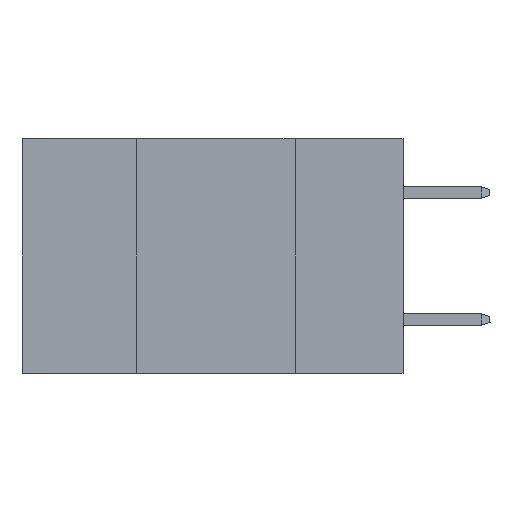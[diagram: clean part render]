
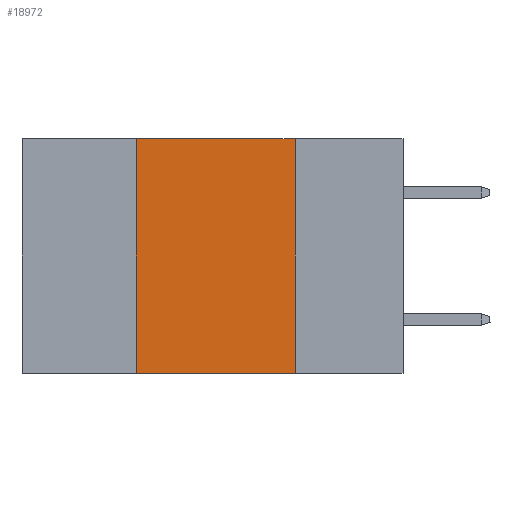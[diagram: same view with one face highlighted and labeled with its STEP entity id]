
A CAD part, left-side view. The second image highlights one B-rep face of the part: STEP entity #18972.
In plain terms, the highlighted planar face has unit normal (-1, 0, 0).
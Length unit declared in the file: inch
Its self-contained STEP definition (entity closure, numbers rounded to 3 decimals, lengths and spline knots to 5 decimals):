
#32 = FACE_OUTER_BOUND ( 'NONE', #22757, .T. ) ;
#1107 = LINE ( 'NONE', #20510, #4530 ) ;
#1899 = VECTOR ( 'NONE', #18962, 39.37008 ) ;
#3018 = VERTEX_POINT ( 'NONE', #8340 ) ;
#3352 = DIRECTION ( 'NONE',  ( 0., 0., 1. ) ) ;
#3910 = PLANE ( 'NONE',  #14600 ) ;
#4316 = ORIENTED_EDGE ( 'NONE', *, *, #20041, .F. ) ;
#4329 = ORIENTED_EDGE ( 'NONE', *, *, #23785, .F. ) ;
#4530 = VECTOR ( 'NONE', #3352, 39.37008 ) ;
#4694 = ORIENTED_EDGE ( 'NONE', *, *, #9097, .T. ) ;
#5408 = VERTEX_POINT ( 'NONE', #8765 ) ;
#5969 = LINE ( 'NONE', #8219, #9829 ) ;
#6471 = EDGE_CURVE ( 'NONE', #5408, #3018, #1107, .T. ) ;
#7242 = VECTOR ( 'NONE', #10525, 39.37008 ) ;
#7670 = CARTESIAN_POINT ( 'NONE',  ( 0., 0.6, 0. ) ) ;
#8219 = CARTESIAN_POINT ( 'NONE',  ( 0., 0.6, 0. ) ) ;
#8340 = CARTESIAN_POINT ( 'NONE',  ( 0., 0.42, 0. ) ) ;
#8765 = CARTESIAN_POINT ( 'NONE',  ( 0., 0.42, -0.37 ) ) ;
#8882 = LINE ( 'NONE', #12286, #7242 ) ;
#9097 = EDGE_CURVE ( 'NONE', #5408, #13345, #8882, .T. ) ;
#9291 = LINE ( 'NONE', #24577, #1899 ) ;
#9829 = VECTOR ( 'NONE', #21253, 39.37008 ) ;
#10131 = CARTESIAN_POINT ( 'NONE',  ( 0., 0.17, -0.37 ) ) ;
#10525 = DIRECTION ( 'NONE',  ( 0., -1., 0. ) ) ;
#10665 = ORIENTED_EDGE ( 'NONE', *, *, #6471, .F. ) ;
#12286 = CARTESIAN_POINT ( 'NONE',  ( 0., 0.6, -0.37 ) ) ;
#13345 = VERTEX_POINT ( 'NONE', #10131 ) ;
#14424 = CARTESIAN_POINT ( 'NONE',  ( 0., 0.17, 0. ) ) ;
#14577 = VERTEX_POINT ( 'NONE', #14424 ) ;
#14600 = AXIS2_PLACEMENT_3D ( 'NONE', #7670, #23072, #15350 ) ;
#15350 = DIRECTION ( 'NONE',  ( 0., 0., -1. ) ) ;
#18962 = DIRECTION ( 'NONE',  ( 0., 0., -1. ) ) ;
#18972 = ADVANCED_FACE ( 'NONE', ( #32 ), #3910, .F. ) ;
#20041 = EDGE_CURVE ( 'NONE', #3018, #14577, #5969, .T. ) ;
#20510 = CARTESIAN_POINT ( 'NONE',  ( 0., 0.42, 0. ) ) ;
#21253 = DIRECTION ( 'NONE',  ( 0., -1., 0. ) ) ;
#22757 = EDGE_LOOP ( 'NONE', ( #4329, #4316, #10665, #4694 ) ) ;
#23072 = DIRECTION ( 'NONE',  ( 1., 0., 0. ) ) ;
#23785 = EDGE_CURVE ( 'NONE', #14577, #13345, #9291, .T. ) ;
#24577 = CARTESIAN_POINT ( 'NONE',  ( 0., 0.17, 0. ) ) ;
